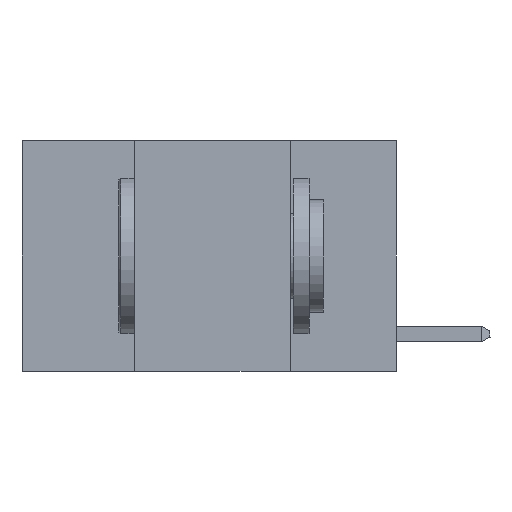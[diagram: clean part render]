
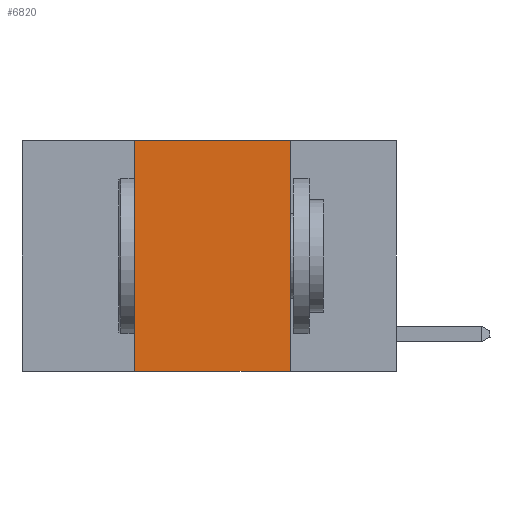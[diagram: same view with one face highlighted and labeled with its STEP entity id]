
A CAD part, left-side view. The second image highlights one B-rep face of the part: STEP entity #6820.
In plain terms, the highlighted planar face has unit normal (-1, 0, 0).
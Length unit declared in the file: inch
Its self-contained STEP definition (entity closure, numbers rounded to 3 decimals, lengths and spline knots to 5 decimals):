
#975 = CARTESIAN_POINT ( 'NONE',  ( 0., 0.17, 0. ) ) ;
#1041 = ORIENTED_EDGE ( 'NONE', *, *, #4018, .F. ) ;
#1114 = EDGE_CURVE ( 'NONE', #3086, #2594, #6599, .T. ) ;
#1119 = CARTESIAN_POINT ( 'NONE',  ( 0., 0.17, 0. ) ) ;
#1796 = DIRECTION ( 'NONE',  ( 0., 0., 1. ) ) ;
#2240 = EDGE_CURVE ( 'NONE', #5692, #3714, #8487, .T. ) ;
#2594 = VERTEX_POINT ( 'NONE', #4516 ) ;
#3086 = VERTEX_POINT ( 'NONE', #12369 ) ;
#3714 = VERTEX_POINT ( 'NONE', #1119 ) ;
#4018 = EDGE_CURVE ( 'NONE', #3714, #2594, #8925, .T. ) ;
#4443 = FACE_OUTER_BOUND ( 'NONE', #9242, .T. ) ;
#4516 = CARTESIAN_POINT ( 'NONE',  ( 0., 0.17, -0.37 ) ) ;
#4760 = CARTESIAN_POINT ( 'NONE',  ( 0., 0.42, 0. ) ) ;
#5225 = ORIENTED_EDGE ( 'NONE', *, *, #2240, .F. ) ;
#5692 = VERTEX_POINT ( 'NONE', #7719 ) ;
#5791 = VECTOR ( 'NONE', #11611, 39.37008 ) ;
#6330 = CARTESIAN_POINT ( 'NONE',  ( 0., 0.6, 0. ) ) ;
#6371 = ORIENTED_EDGE ( 'NONE', *, *, #1114, .T. ) ;
#6599 = LINE ( 'NONE', #10535, #7821 ) ;
#6820 = ADVANCED_FACE ( 'NONE', ( #4443 ), #7541, .F. ) ;
#7320 = VECTOR ( 'NONE', #1796, 39.37008 ) ;
#7541 = PLANE ( 'NONE',  #8471 ) ;
#7719 = CARTESIAN_POINT ( 'NONE',  ( 0., 0.42, 0. ) ) ;
#7821 = VECTOR ( 'NONE', #9766, 39.37008 ) ;
#8471 = AXIS2_PLACEMENT_3D ( 'NONE', #6330, #8480, #10266 ) ;
#8480 = DIRECTION ( 'NONE',  ( 1., 0., 0. ) ) ;
#8487 = LINE ( 'NONE', #8749, #5791 ) ;
#8564 = VECTOR ( 'NONE', #8798, 39.37008 ) ;
#8749 = CARTESIAN_POINT ( 'NONE',  ( 0., 0.6, 0. ) ) ;
#8798 = DIRECTION ( 'NONE',  ( 0., 0., -1. ) ) ;
#8925 = LINE ( 'NONE', #975, #8564 ) ;
#9242 = EDGE_LOOP ( 'NONE', ( #1041, #5225, #9383, #6371 ) ) ;
#9383 = ORIENTED_EDGE ( 'NONE', *, *, #9932, .F. ) ;
#9766 = DIRECTION ( 'NONE',  ( 0., -1., 0. ) ) ;
#9932 = EDGE_CURVE ( 'NONE', #3086, #5692, #10719, .T. ) ;
#10266 = DIRECTION ( 'NONE',  ( 0., 0., -1. ) ) ;
#10535 = CARTESIAN_POINT ( 'NONE',  ( 0., 0.6, -0.37 ) ) ;
#10719 = LINE ( 'NONE', #4760, #7320 ) ;
#11611 = DIRECTION ( 'NONE',  ( 0., -1., 0. ) ) ;
#12369 = CARTESIAN_POINT ( 'NONE',  ( 0., 0.42, -0.37 ) ) ;
